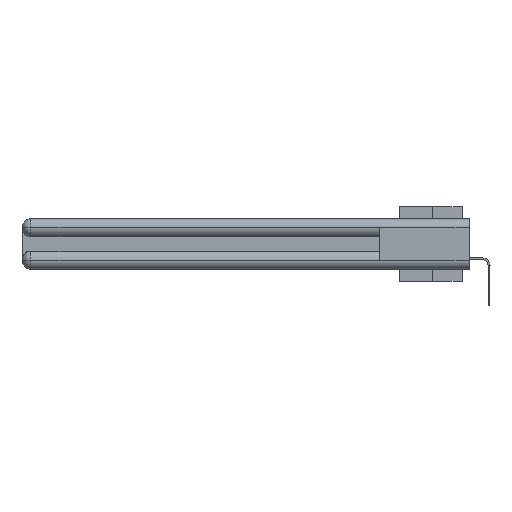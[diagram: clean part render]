
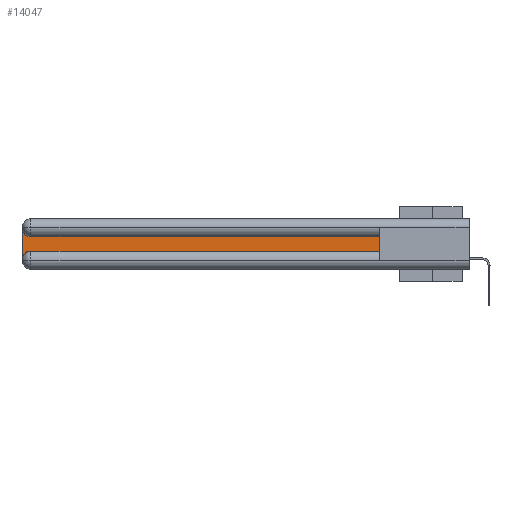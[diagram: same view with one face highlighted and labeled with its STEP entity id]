
A CAD part, left-side view. The second image highlights one B-rep face of the part: STEP entity #14047.
In plain terms, the highlighted planar face has unit normal (-1, 0, 0).
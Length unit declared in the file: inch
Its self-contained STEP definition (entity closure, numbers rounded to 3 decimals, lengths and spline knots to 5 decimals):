
#2262 = VECTOR ( 'NONE', #24936, 39.37008 ) ;
#3292 = AXIS2_PLACEMENT_3D ( 'NONE', #3991, #31642, #14237 ) ;
#3322 = ORIENTED_EDGE ( 'NONE', *, *, #12592, .T. ) ;
#3369 = CARTESIAN_POINT ( 'NONE',  ( 0.075, 3., -0.2175 ) ) ;
#3991 = CARTESIAN_POINT ( 'NONE',  ( 0.075, 2.94, -0.0625 ) ) ;
#4274 = VERTEX_POINT ( 'NONE', #14985 ) ;
#4564 = DIRECTION ( 'NONE',  ( 1., 0., 0. ) ) ;
#5312 = DIRECTION ( 'NONE',  ( 0., 1., 0. ) ) ;
#5388 = DIRECTION ( 'NONE',  ( 0., 0., -1. ) ) ;
#5781 = ORIENTED_EDGE ( 'NONE', *, *, #6018, .T. ) ;
#6018 = EDGE_CURVE ( 'NONE', #7408, #21426, #30527, .T. ) ;
#7014 = PLANE ( 'NONE',  #10506 ) ;
#7042 = LINE ( 'NONE', #13489, #28120 ) ;
#7408 = VERTEX_POINT ( 'NONE', #31770 ) ;
#8039 = DIRECTION ( 'NONE',  ( 1., 0., 0. ) ) ;
#9686 = DIRECTION ( 'NONE',  ( 0., 0., -1. ) ) ;
#9855 = ORIENTED_EDGE ( 'NONE', *, *, #28187, .T. ) ;
#10141 = EDGE_CURVE ( 'NONE', #21426, #21185, #13165, .T. ) ;
#10192 = CARTESIAN_POINT ( 'NONE',  ( 0.075, 0.6, -0.1225 ) ) ;
#10417 = VECTOR ( 'NONE', #25856, 39.37008 ) ;
#10506 = AXIS2_PLACEMENT_3D ( 'NONE', #12108, #4564, #9686 ) ;
#12108 = CARTESIAN_POINT ( 'NONE',  ( 0.075, 3., -0.1225 ) ) ;
#12592 = EDGE_CURVE ( 'NONE', #12630, #7408, #12895, .T. ) ;
#12630 = VERTEX_POINT ( 'NONE', #20435 ) ;
#12895 = LINE ( 'NONE', #10192, #28441 ) ;
#13165 = LINE ( 'NONE', #3369, #10417 ) ;
#13244 = EDGE_LOOP ( 'NONE', ( #3322, #5781, #32403, #26924, #16417, #9855 ) ) ;
#13489 = CARTESIAN_POINT ( 'NONE',  ( 0.075, 0.6, -0.2175 ) ) ;
#14047 = ADVANCED_FACE ( 'NONE', ( #31075 ), #7014, .F. ) ;
#14237 = DIRECTION ( 'NONE',  ( 0., 0., -1. ) ) ;
#14267 = CIRCLE ( 'NONE', #26971, 0.06 ) ;
#14985 = CARTESIAN_POINT ( 'NONE',  ( 0.075, 2.94, -0.2175 ) ) ;
#15518 = CARTESIAN_POINT ( 'NONE',  ( 0.075, 3., -0.0625 ) ) ;
#16074 = DIRECTION ( 'NONE',  ( 0., 0., 1. ) ) ;
#16292 = EDGE_CURVE ( 'NONE', #21185, #4274, #14267, .T. ) ;
#16417 = ORIENTED_EDGE ( 'NONE', *, *, #19921, .T. ) ;
#19921 = EDGE_CURVE ( 'NONE', #4274, #28960, #24528, .T. ) ;
#19927 = CARTESIAN_POINT ( 'NONE',  ( 0.075, 0.6, -0.2175 ) ) ;
#20435 = CARTESIAN_POINT ( 'NONE',  ( 0.075, 0.6, -0.1225 ) ) ;
#21185 = VERTEX_POINT ( 'NONE', #27413 ) ;
#21426 = VERTEX_POINT ( 'NONE', #15518 ) ;
#22271 = CARTESIAN_POINT ( 'NONE',  ( 0.075, 0.6, -0.2175 ) ) ;
#23071 = CARTESIAN_POINT ( 'NONE',  ( 0.075, 2.94, -0.2775 ) ) ;
#24528 = LINE ( 'NONE', #19927, #2262 ) ;
#24936 = DIRECTION ( 'NONE',  ( 0., -1., 0. ) ) ;
#25856 = DIRECTION ( 'NONE',  ( 0., 0., -1. ) ) ;
#26924 = ORIENTED_EDGE ( 'NONE', *, *, #16292, .T. ) ;
#26971 = AXIS2_PLACEMENT_3D ( 'NONE', #23071, #8039, #5388 ) ;
#27413 = CARTESIAN_POINT ( 'NONE',  ( 0.075, 3., -0.2775 ) ) ;
#28120 = VECTOR ( 'NONE', #16074, 39.37008 ) ;
#28187 = EDGE_CURVE ( 'NONE', #28960, #12630, #7042, .T. ) ;
#28441 = VECTOR ( 'NONE', #5312, 39.37008 ) ;
#28960 = VERTEX_POINT ( 'NONE', #22271 ) ;
#30527 = CIRCLE ( 'NONE', #3292, 0.06 ) ;
#31075 = FACE_OUTER_BOUND ( 'NONE', #13244, .T. ) ;
#31642 = DIRECTION ( 'NONE',  ( 1., 0., 0. ) ) ;
#31770 = CARTESIAN_POINT ( 'NONE',  ( 0.075, 2.94, -0.1225 ) ) ;
#32403 = ORIENTED_EDGE ( 'NONE', *, *, #10141, .T. ) ;
